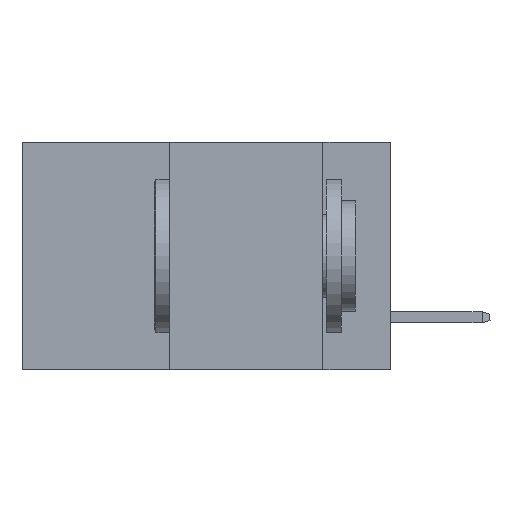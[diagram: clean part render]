
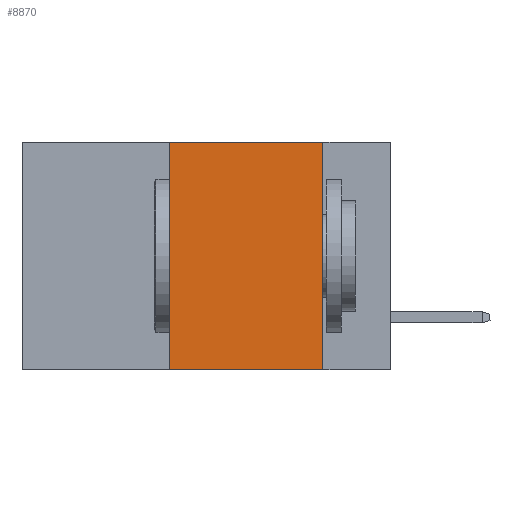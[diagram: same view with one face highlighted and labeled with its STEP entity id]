
A CAD part, left-side view. The second image highlights one B-rep face of the part: STEP entity #8870.
In plain terms, the highlighted planar face has unit normal (-1, 0, 0).
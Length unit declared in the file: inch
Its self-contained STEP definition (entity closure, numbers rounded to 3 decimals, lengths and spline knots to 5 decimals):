
#47 = PLANE ( 'NONE',  #5712 ) ;
#96 = LINE ( 'NONE', #11261, #6081 ) ;
#390 = CARTESIAN_POINT ( 'NONE',  ( 0., 0.6, 0. ) ) ;
#491 = LINE ( 'NONE', #6199, #11303 ) ;
#548 = EDGE_CURVE ( 'NONE', #8817, #7260, #96, .T. ) ;
#693 = EDGE_CURVE ( 'NONE', #2974, #11072, #5947, .T. ) ;
#1227 = EDGE_LOOP ( 'NONE', ( #5828, #9962, #5375, #6259 ) ) ;
#1523 = FACE_OUTER_BOUND ( 'NONE', #1227, .T. ) ;
#2664 = CARTESIAN_POINT ( 'NONE',  ( 0., 0.36, 0. ) ) ;
#2974 = VERTEX_POINT ( 'NONE', #3674 ) ;
#3116 = CARTESIAN_POINT ( 'NONE',  ( 0., 0.11, 0. ) ) ;
#3454 = DIRECTION ( 'NONE',  ( 0., 0., -1. ) ) ;
#3674 = CARTESIAN_POINT ( 'NONE',  ( 0., 0.36, 0. ) ) ;
#3769 = CARTESIAN_POINT ( 'NONE',  ( 0., 0.11, -0.37 ) ) ;
#3857 = CARTESIAN_POINT ( 'NONE',  ( 0., 0.6, 0. ) ) ;
#3974 = VECTOR ( 'NONE', #7420, 39.37008 ) ;
#4136 = DIRECTION ( 'NONE',  ( 0., -1., 0. ) ) ;
#4609 = CARTESIAN_POINT ( 'NONE',  ( 0., 0.36, -0.37 ) ) ;
#5005 = EDGE_CURVE ( 'NONE', #11072, #7260, #491, .T. ) ;
#5375 = ORIENTED_EDGE ( 'NONE', *, *, #6179, .F. ) ;
#5712 = AXIS2_PLACEMENT_3D ( 'NONE', #3857, #6531, #10954 ) ;
#5828 = ORIENTED_EDGE ( 'NONE', *, *, #5005, .F. ) ;
#5947 = LINE ( 'NONE', #390, #3974 ) ;
#6081 = VECTOR ( 'NONE', #4136, 39.37008 ) ;
#6179 = EDGE_CURVE ( 'NONE', #8817, #2974, #6192, .T. ) ;
#6192 = LINE ( 'NONE', #2664, #9088 ) ;
#6199 = CARTESIAN_POINT ( 'NONE',  ( 0., 0.11, 0. ) ) ;
#6259 = ORIENTED_EDGE ( 'NONE', *, *, #548, .T. ) ;
#6531 = DIRECTION ( 'NONE',  ( 1., 0., 0. ) ) ;
#7260 = VERTEX_POINT ( 'NONE', #3769 ) ;
#7420 = DIRECTION ( 'NONE',  ( 0., -1., 0. ) ) ;
#8742 = DIRECTION ( 'NONE',  ( 0., 0., 1. ) ) ;
#8817 = VERTEX_POINT ( 'NONE', #4609 ) ;
#8870 = ADVANCED_FACE ( 'NONE', ( #1523 ), #47, .F. ) ;
#9088 = VECTOR ( 'NONE', #8742, 39.37008 ) ;
#9962 = ORIENTED_EDGE ( 'NONE', *, *, #693, .F. ) ;
#10954 = DIRECTION ( 'NONE',  ( 0., 0., -1. ) ) ;
#11072 = VERTEX_POINT ( 'NONE', #3116 ) ;
#11261 = CARTESIAN_POINT ( 'NONE',  ( 0., 0.6, -0.37 ) ) ;
#11303 = VECTOR ( 'NONE', #3454, 39.37008 ) ;
